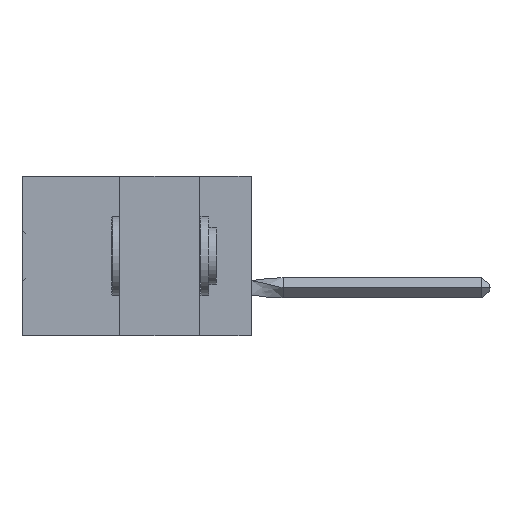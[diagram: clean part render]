
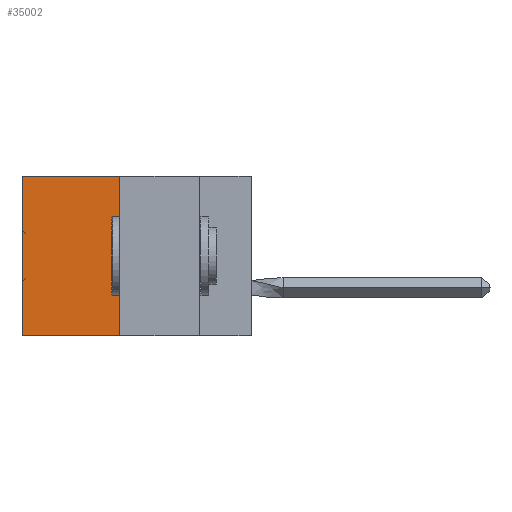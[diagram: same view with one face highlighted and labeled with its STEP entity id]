
A CAD part, left-side view. The second image highlights one B-rep face of the part: STEP entity #35002.
In plain terms, the highlighted planar face has unit normal (-1, 0, 0).
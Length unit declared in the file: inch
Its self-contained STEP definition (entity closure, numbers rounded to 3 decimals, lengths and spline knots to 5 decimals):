
#1908 = ORIENTED_EDGE ( 'NONE', *, *, #36789, .F. ) ;
#3322 = DIRECTION ( 'NONE',  ( 0., 1., 0. ) ) ;
#3800 = EDGE_CURVE ( 'NONE', #5872, #49813, #57134, .T. ) ;
#4133 = CARTESIAN_POINT ( 'NONE',  ( 0.305, 0.413, -0.5 ) ) ;
#4689 = CARTESIAN_POINT ( 'NONE',  ( 0.305, 0.72, 0. ) ) ;
#5048 = CARTESIAN_POINT ( 'NONE',  ( 0.305, 0.413, -0.5 ) ) ;
#5872 = VERTEX_POINT ( 'NONE', #4689 ) ;
#8510 = DIRECTION ( 'NONE',  ( 1., 0., 0. ) ) ;
#9544 = EDGE_CURVE ( 'NONE', #53142, #5872, #48399, .T. ) ;
#13161 = EDGE_CURVE ( 'NONE', #53142, #17321, #14554, .T. ) ;
#14554 = LINE ( 'NONE', #56247, #35112 ) ;
#17321 = VERTEX_POINT ( 'NONE', #5048 ) ;
#21894 = CARTESIAN_POINT ( 'NONE',  ( 0.305, 0.72, -0.5 ) ) ;
#22482 = PLANE ( 'NONE',  #41782 ) ;
#23377 = FACE_OUTER_BOUND ( 'NONE', #25732, .T. ) ;
#23410 = CARTESIAN_POINT ( 'NONE',  ( 0.305, 0.413, 0. ) ) ;
#23485 = ORIENTED_EDGE ( 'NONE', *, *, #9544, .T. ) ;
#23522 = DIRECTION ( 'NONE',  ( 0., 1., 0. ) ) ;
#24665 = LINE ( 'NONE', #41875, #35252 ) ;
#25732 = EDGE_LOOP ( 'NONE', ( #42892, #1908, #58189, #23485 ) ) ;
#25740 = VECTOR ( 'NONE', #3322, 39.37008 ) ;
#29415 = VECTOR ( 'NONE', #48701, 39.37008 ) ;
#35002 = ADVANCED_FACE ( 'NONE', ( #23377 ), #22482, .F. ) ;
#35112 = VECTOR ( 'NONE', #42062, 39.37008 ) ;
#35252 = VECTOR ( 'NONE', #23522, 39.37008 ) ;
#36789 = EDGE_CURVE ( 'NONE', #17321, #49813, #24665, .T. ) ;
#41782 = AXIS2_PLACEMENT_3D ( 'NONE', #4133, #8510, #54267 ) ;
#41875 = CARTESIAN_POINT ( 'NONE',  ( 0.305, 0.413, -0.5 ) ) ;
#42062 = DIRECTION ( 'NONE',  ( 0., 0., -1. ) ) ;
#42892 = ORIENTED_EDGE ( 'NONE', *, *, #3800, .T. ) ;
#43727 = CARTESIAN_POINT ( 'NONE',  ( 0.305, 0.72, -0.5 ) ) ;
#48399 = LINE ( 'NONE', #53436, #25740 ) ;
#48701 = DIRECTION ( 'NONE',  ( 0., 0., -1. ) ) ;
#49813 = VERTEX_POINT ( 'NONE', #43727 ) ;
#53142 = VERTEX_POINT ( 'NONE', #23410 ) ;
#53436 = CARTESIAN_POINT ( 'NONE',  ( 0.305, 0.413, 0. ) ) ;
#54267 = DIRECTION ( 'NONE',  ( 0., 0., -1. ) ) ;
#56247 = CARTESIAN_POINT ( 'NONE',  ( 0.305, 0.413, -0.5 ) ) ;
#57134 = LINE ( 'NONE', #21894, #29415 ) ;
#58189 = ORIENTED_EDGE ( 'NONE', *, *, #13161, .F. ) ;
